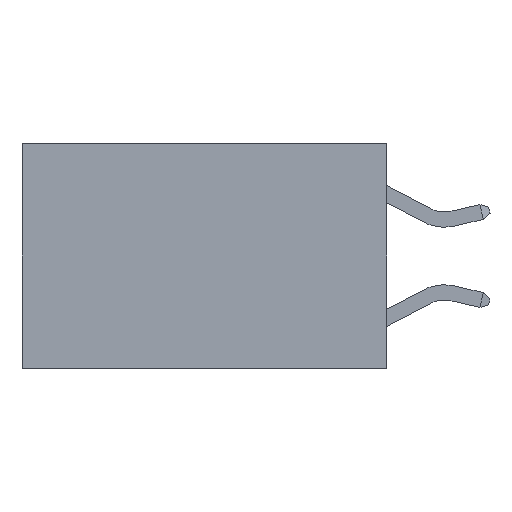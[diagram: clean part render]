
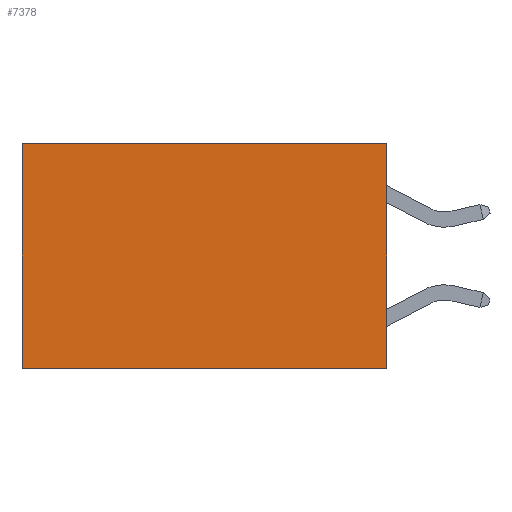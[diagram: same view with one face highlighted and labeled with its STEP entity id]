
A CAD part, left-side view. The second image highlights one B-rep face of the part: STEP entity #7378.
In plain terms, the highlighted planar face has unit normal (-1, 0, 0).
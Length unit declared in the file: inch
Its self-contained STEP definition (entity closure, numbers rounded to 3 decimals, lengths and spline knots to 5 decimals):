
#3147 = CARTESIAN_POINT ( 'NONE',  ( 0.2625, 0., 0. ) ) ;
#7378 = ADVANCED_FACE ( 'NONE', ( #28692 ), #12887, .F. ) ;
#7679 = ORIENTED_EDGE ( 'NONE', *, *, #10563, .T. ) ;
#8234 = EDGE_CURVE ( 'NONE', #23933, #22451, #17636, .T. ) ;
#8565 = AXIS2_PLACEMENT_3D ( 'NONE', #3147, #29894, #22666 ) ;
#10335 = VERTEX_POINT ( 'NONE', #14748 ) ;
#10563 = EDGE_CURVE ( 'NONE', #23933, #10335, #16317, .T. ) ;
#10973 = DIRECTION ( 'NONE',  ( 0., 0., -1. ) ) ;
#11202 = DIRECTION ( 'NONE',  ( 0., 1., 0. ) ) ;
#12448 = CARTESIAN_POINT ( 'NONE',  ( 0.2625, 0., -0.37 ) ) ;
#12887 = PLANE ( 'NONE',  #8565 ) ;
#13869 = DIRECTION ( 'NONE',  ( 0., 0., -1. ) ) ;
#14370 = VERTEX_POINT ( 'NONE', #29678 ) ;
#14748 = CARTESIAN_POINT ( 'NONE',  ( 0.2625, 0.6, 0. ) ) ;
#14764 = CARTESIAN_POINT ( 'NONE',  ( 0.2625, 0., 0. ) ) ;
#14776 = ORIENTED_EDGE ( 'NONE', *, *, #8234, .F. ) ;
#16010 = VECTOR ( 'NONE', #13869, 39.37008 ) ;
#16317 = LINE ( 'NONE', #20323, #18979 ) ;
#17503 = LINE ( 'NONE', #28510, #16010 ) ;
#17636 = LINE ( 'NONE', #20637, #20272 ) ;
#18979 = VECTOR ( 'NONE', #11202, 39.37008 ) ;
#19230 = EDGE_LOOP ( 'NONE', ( #25893, #25221, #14776, #7679 ) ) ;
#20272 = VECTOR ( 'NONE', #10973, 39.37008 ) ;
#20323 = CARTESIAN_POINT ( 'NONE',  ( 0.2625, 0., 0. ) ) ;
#20637 = CARTESIAN_POINT ( 'NONE',  ( 0.2625, 0., 0. ) ) ;
#22451 = VERTEX_POINT ( 'NONE', #12448 ) ;
#22643 = VECTOR ( 'NONE', #30266, 39.37008 ) ;
#22666 = DIRECTION ( 'NONE',  ( 0., 0., -1. ) ) ;
#23150 = CARTESIAN_POINT ( 'NONE',  ( 0.2625, 0., -0.37 ) ) ;
#23933 = VERTEX_POINT ( 'NONE', #14764 ) ;
#24107 = EDGE_CURVE ( 'NONE', #22451, #14370, #28703, .T. ) ;
#25221 = ORIENTED_EDGE ( 'NONE', *, *, #24107, .F. ) ;
#25893 = ORIENTED_EDGE ( 'NONE', *, *, #31286, .T. ) ;
#28510 = CARTESIAN_POINT ( 'NONE',  ( 0.2625, 0.6, 0. ) ) ;
#28692 = FACE_OUTER_BOUND ( 'NONE', #19230, .T. ) ;
#28703 = LINE ( 'NONE', #23150, #22643 ) ;
#29678 = CARTESIAN_POINT ( 'NONE',  ( 0.2625, 0.6, -0.37 ) ) ;
#29894 = DIRECTION ( 'NONE',  ( 1., 0., 0. ) ) ;
#30266 = DIRECTION ( 'NONE',  ( 0., 1., 0. ) ) ;
#31286 = EDGE_CURVE ( 'NONE', #10335, #14370, #17503, .T. ) ;
